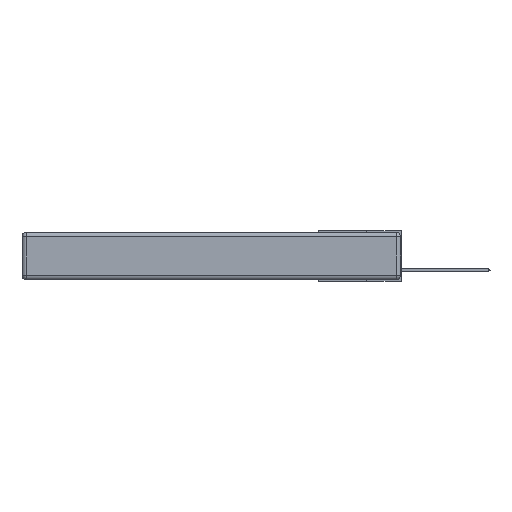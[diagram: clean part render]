
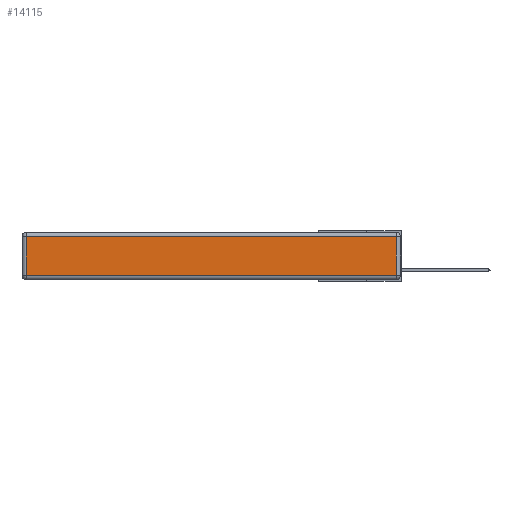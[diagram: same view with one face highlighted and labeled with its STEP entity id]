
A CAD part, left-side view. The second image highlights one B-rep face of the part: STEP entity #14115.
In plain terms, the highlighted planar face has unit normal (-1, 0, 0).
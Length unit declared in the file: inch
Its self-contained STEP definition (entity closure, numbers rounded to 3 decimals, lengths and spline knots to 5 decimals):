
#874 = EDGE_LOOP ( 'NONE', ( #1611, #21096, #24996, #24924 ) ) ;
#990 = LINE ( 'NONE', #21651, #21495 ) ;
#1305 = VECTOR ( 'NONE', #15087, 39.37008 ) ;
#1611 = ORIENTED_EDGE ( 'NONE', *, *, #14674, .T. ) ;
#1857 = DIRECTION ( 'NONE',  ( -1., 0., 0. ) ) ;
#2627 = VECTOR ( 'NONE', #24644, 39.37008 ) ;
#3108 = DIRECTION ( 'NONE',  ( 0., 0., 1. ) ) ;
#4151 = CARTESIAN_POINT ( 'NONE',  ( 0., 2.72, -0.03 ) ) ;
#5665 = LINE ( 'NONE', #19139, #1305 ) ;
#6162 = DIRECTION ( 'NONE',  ( 0., 0., 1. ) ) ;
#8083 = FACE_OUTER_BOUND ( 'NONE', #874, .T. ) ;
#10259 = VERTEX_POINT ( 'NONE', #11599 ) ;
#10395 = LINE ( 'NONE', #15802, #11423 ) ;
#10473 = CARTESIAN_POINT ( 'NONE',  ( 0., 0., -0.343 ) ) ;
#11423 = VECTOR ( 'NONE', #3108, 39.37008 ) ;
#11599 = CARTESIAN_POINT ( 'NONE',  ( 0., 0.03, -0.313 ) ) ;
#12766 = EDGE_CURVE ( 'NONE', #10259, #24254, #10395, .T. ) ;
#13787 = VERTEX_POINT ( 'NONE', #23995 ) ;
#14073 = EDGE_CURVE ( 'NONE', #24254, #18357, #25805, .T. ) ;
#14115 = ADVANCED_FACE ( 'NONE', ( #8083 ), #19016, .T. ) ;
#14346 = EDGE_CURVE ( 'NONE', #18357, #13787, #990, .T. ) ;
#14674 = EDGE_CURVE ( 'NONE', #13787, #10259, #5665, .T. ) ;
#15087 = DIRECTION ( 'NONE',  ( 0., -1., 0. ) ) ;
#15802 = CARTESIAN_POINT ( 'NONE',  ( 0., 0.03, -0.343 ) ) ;
#17548 = AXIS2_PLACEMENT_3D ( 'NONE', #10473, #1857, #6162 ) ;
#18357 = VERTEX_POINT ( 'NONE', #4151 ) ;
#18399 = CARTESIAN_POINT ( 'NONE',  ( 0., 2.75, -0.03 ) ) ;
#18951 = CARTESIAN_POINT ( 'NONE',  ( 0., 0.03, -0.03 ) ) ;
#19016 = PLANE ( 'NONE',  #17548 ) ;
#19139 = CARTESIAN_POINT ( 'NONE',  ( 0., 0., -0.313 ) ) ;
#21096 = ORIENTED_EDGE ( 'NONE', *, *, #12766, .T. ) ;
#21495 = VECTOR ( 'NONE', #21855, 39.37008 ) ;
#21651 = CARTESIAN_POINT ( 'NONE',  ( 0., 2.72, -0.343 ) ) ;
#21855 = DIRECTION ( 'NONE',  ( 0., 0., -1. ) ) ;
#23995 = CARTESIAN_POINT ( 'NONE',  ( 0., 2.72, -0.313 ) ) ;
#24254 = VERTEX_POINT ( 'NONE', #18951 ) ;
#24644 = DIRECTION ( 'NONE',  ( 0., 1., 0. ) ) ;
#24924 = ORIENTED_EDGE ( 'NONE', *, *, #14346, .T. ) ;
#24996 = ORIENTED_EDGE ( 'NONE', *, *, #14073, .T. ) ;
#25805 = LINE ( 'NONE', #18399, #2627 ) ;
